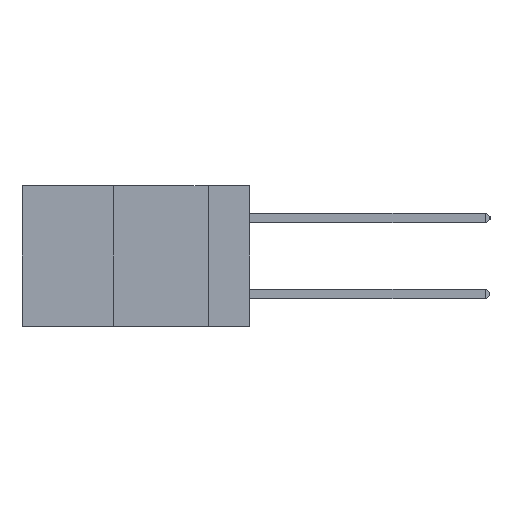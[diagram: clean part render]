
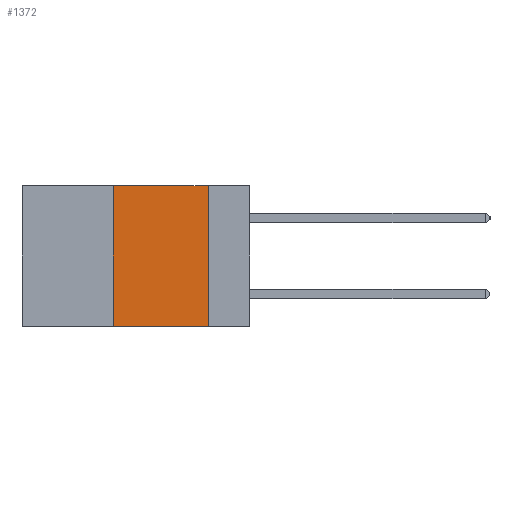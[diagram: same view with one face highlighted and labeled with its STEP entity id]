
A CAD part, left-side view. The second image highlights one B-rep face of the part: STEP entity #1372.
In plain terms, the highlighted planar face has unit normal (-1, 0, 0).
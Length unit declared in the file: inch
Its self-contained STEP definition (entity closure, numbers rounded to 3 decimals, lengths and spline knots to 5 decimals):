
#429 = ORIENTED_EDGE ( 'NONE', *, *, #4013, .F. ) ;
#916 = PLANE ( 'NONE',  #8142 ) ;
#1372 = ADVANCED_FACE ( 'NONE', ( #5241 ), #916, .F. ) ;
#1438 = CARTESIAN_POINT ( 'NONE',  ( 0., 0.36, 0. ) ) ;
#1779 = CARTESIAN_POINT ( 'NONE',  ( 0., 0.6, 0. ) ) ;
#2150 = LINE ( 'NONE', #9535, #6852 ) ;
#3127 = VECTOR ( 'NONE', #5030, 39.37008 ) ;
#3486 = VERTEX_POINT ( 'NONE', #4373 ) ;
#4013 = EDGE_CURVE ( 'NONE', #8492, #8532, #10491, .T. ) ;
#4193 = DIRECTION ( 'NONE',  ( 0., 0., -1. ) ) ;
#4248 = VECTOR ( 'NONE', #5499, 39.37008 ) ;
#4373 = CARTESIAN_POINT ( 'NONE',  ( 0., 0.11, -0.37 ) ) ;
#4524 = VERTEX_POINT ( 'NONE', #6538 ) ;
#4878 = DIRECTION ( 'NONE',  ( 0., 0., -1. ) ) ;
#5030 = DIRECTION ( 'NONE',  ( 0., 0., 1. ) ) ;
#5241 = FACE_OUTER_BOUND ( 'NONE', #6486, .T. ) ;
#5499 = DIRECTION ( 'NONE',  ( 0., -1., 0. ) ) ;
#5688 = DIRECTION ( 'NONE',  ( 0., -1., 0. ) ) ;
#6410 = CARTESIAN_POINT ( 'NONE',  ( 0., 0.6, -0.37 ) ) ;
#6486 = EDGE_LOOP ( 'NONE', ( #8679, #7106, #429, #9766 ) ) ;
#6538 = CARTESIAN_POINT ( 'NONE',  ( 0., 0.11, 0. ) ) ;
#6822 = EDGE_CURVE ( 'NONE', #4524, #3486, #2150, .T. ) ;
#6852 = VECTOR ( 'NONE', #4193, 39.37008 ) ;
#7011 = CARTESIAN_POINT ( 'NONE',  ( 0., 0.36, -0.37 ) ) ;
#7069 = EDGE_CURVE ( 'NONE', #8492, #3486, #9020, .T. ) ;
#7106 = ORIENTED_EDGE ( 'NONE', *, *, #7800, .F. ) ;
#7797 = VECTOR ( 'NONE', #5688, 39.37008 ) ;
#7800 = EDGE_CURVE ( 'NONE', #8532, #4524, #10282, .T. ) ;
#8142 = AXIS2_PLACEMENT_3D ( 'NONE', #1779, #9520, #4878 ) ;
#8300 = CARTESIAN_POINT ( 'NONE',  ( 0., 0.6, 0. ) ) ;
#8343 = CARTESIAN_POINT ( 'NONE',  ( 0., 0.36, 0. ) ) ;
#8492 = VERTEX_POINT ( 'NONE', #7011 ) ;
#8532 = VERTEX_POINT ( 'NONE', #1438 ) ;
#8679 = ORIENTED_EDGE ( 'NONE', *, *, #6822, .F. ) ;
#9020 = LINE ( 'NONE', #6410, #4248 ) ;
#9520 = DIRECTION ( 'NONE',  ( 1., 0., 0. ) ) ;
#9535 = CARTESIAN_POINT ( 'NONE',  ( 0., 0.11, 0. ) ) ;
#9766 = ORIENTED_EDGE ( 'NONE', *, *, #7069, .T. ) ;
#10282 = LINE ( 'NONE', #8300, #7797 ) ;
#10491 = LINE ( 'NONE', #8343, #3127 ) ;
